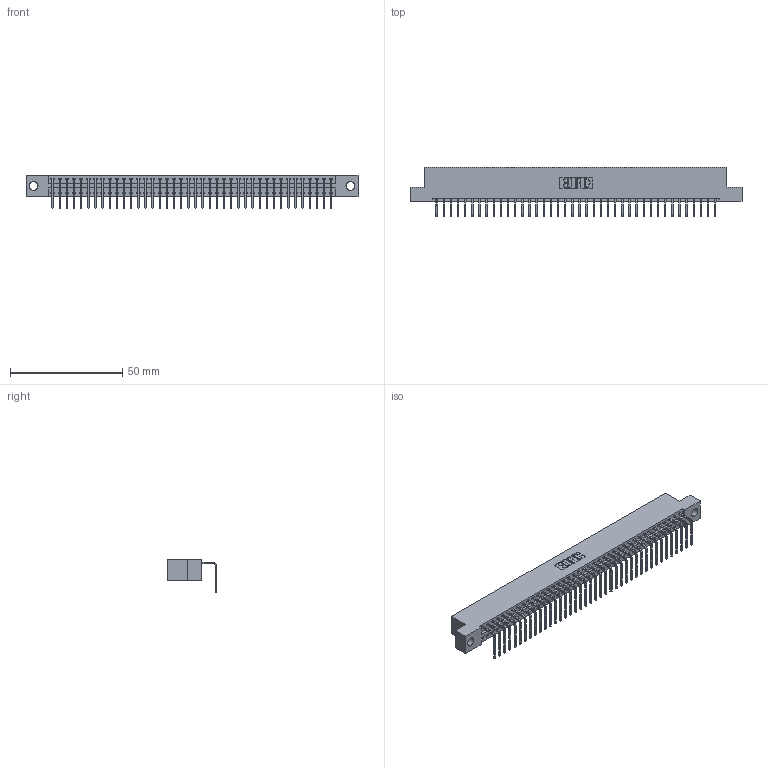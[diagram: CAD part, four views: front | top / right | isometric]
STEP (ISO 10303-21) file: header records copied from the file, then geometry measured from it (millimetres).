
FILE_DESCRIPTION (( 'STEP AP203' ), '1' );
FILE_NAME ('396-040-558-104.STEP', '2018-09-06T21:34:28', ( '' ), ( '' ), 'SwSTEP 2.0', 'SolidWorks 2016', '' );
FILE_SCHEMA (( 'CONFIG_CONTROL_DESIGN' ));
Length unit declared in the file: inch
Products named in the file (3): 396-040-558-104; 346 Part_Flush Mounting Lugs - 0.156 Dia-TH; 345-292-001_558 Tail - 2
Assembly tree (41 placements, depth 2):
  396-040-558-104
    346 Part_Flush Mounting Lugs - 0.156 Dia-TH
    345-292-001_558 Tail - 2  x40
Bounding box: 147.57 x 22.16 x 14.73 mm (x, y, z)
Volume: 14157.7 mm3; surface area: 18273.8 mm2
Topology: 41 solids, 41 shells, 2522 faces, 7609 edges, 5018 vertices
Faces by surface type: plane 1756, cylinder 766
Entity records: 25181 total; most frequent: CARTESIAN_POINT 4324, ORIENTED_EDGE 4298, DIRECTION 3817, EDGE_CURVE 2149, LINE 1857, VECTOR 1857, VERTEX_POINT 1430, AXIS2_PLACEMENT_3D 980
